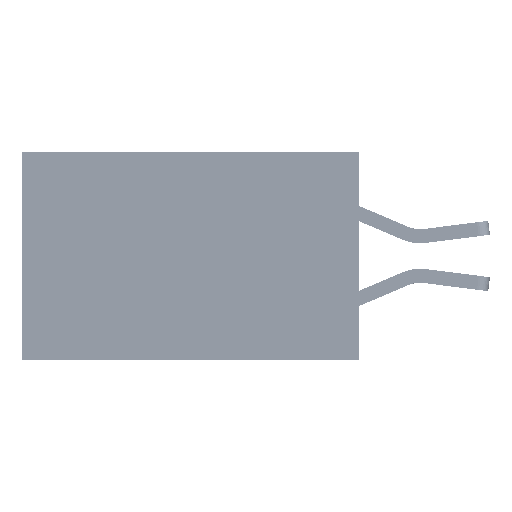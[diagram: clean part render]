
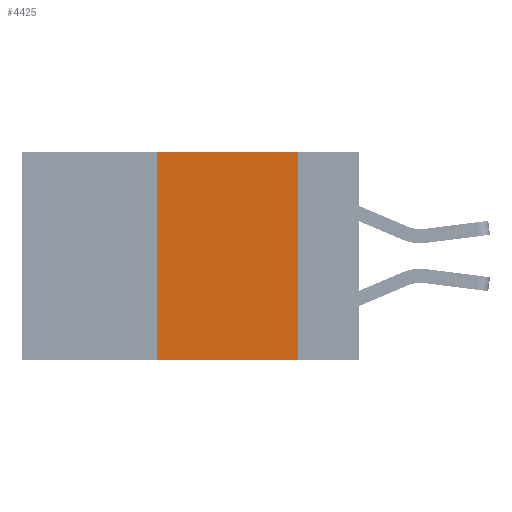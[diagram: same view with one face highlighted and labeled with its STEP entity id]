
A CAD part, left-side view. The second image highlights one B-rep face of the part: STEP entity #4425.
In plain terms, the highlighted planar face has unit normal (-1, 0, 0).
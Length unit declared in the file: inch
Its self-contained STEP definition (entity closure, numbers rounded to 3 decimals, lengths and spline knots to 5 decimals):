
#31 = VERTEX_POINT ( 'NONE', #29388 ) ;
#1272 = CARTESIAN_POINT ( 'NONE',  ( 0., 0.6, -0.37 ) ) ;
#2855 = CARTESIAN_POINT ( 'NONE',  ( 0., 0.6, 0. ) ) ;
#3001 = CARTESIAN_POINT ( 'NONE',  ( 0., 0.11, 0. ) ) ;
#4425 = ADVANCED_FACE ( 'NONE', ( #19435 ), #7295, .F. ) ;
#5041 = VECTOR ( 'NONE', #14315, 39.37008 ) ;
#5146 = VECTOR ( 'NONE', #39077, 39.37008 ) ;
#7295 = PLANE ( 'NONE',  #18443 ) ;
#7898 = EDGE_CURVE ( 'NONE', #31, #11036, #17348, .T. ) ;
#11036 = VERTEX_POINT ( 'NONE', #31494 ) ;
#11077 = ORIENTED_EDGE ( 'NONE', *, *, #44065, .F. ) ;
#12180 = VERTEX_POINT ( 'NONE', #38484 ) ;
#13363 = VERTEX_POINT ( 'NONE', #28481 ) ;
#14315 = DIRECTION ( 'NONE',  ( 0., -1., 0. ) ) ;
#14658 = EDGE_LOOP ( 'NONE', ( #11077, #18350, #37101, #19642 ) ) ;
#14965 = DIRECTION ( 'NONE',  ( 1., 0., 0. ) ) ;
#15253 = LINE ( 'NONE', #2855, #5041 ) ;
#15363 = LINE ( 'NONE', #16987, #5146 ) ;
#16806 = VECTOR ( 'NONE', #18222, 39.37008 ) ;
#16987 = CARTESIAN_POINT ( 'NONE',  ( 0., 0.36, 0. ) ) ;
#17348 = LINE ( 'NONE', #1272, #27207 ) ;
#18222 = DIRECTION ( 'NONE',  ( 0., 0., -1. ) ) ;
#18350 = ORIENTED_EDGE ( 'NONE', *, *, #42104, .F. ) ;
#18443 = AXIS2_PLACEMENT_3D ( 'NONE', #22281, #14965, #40776 ) ;
#19435 = FACE_OUTER_BOUND ( 'NONE', #14658, .T. ) ;
#19642 = ORIENTED_EDGE ( 'NONE', *, *, #7898, .T. ) ;
#21837 = EDGE_CURVE ( 'NONE', #31, #12180, #15363, .T. ) ;
#22281 = CARTESIAN_POINT ( 'NONE',  ( 0., 0.6, 0. ) ) ;
#27207 = VECTOR ( 'NONE', #42366, 39.37008 ) ;
#28481 = CARTESIAN_POINT ( 'NONE',  ( 0., 0.11, 0. ) ) ;
#29388 = CARTESIAN_POINT ( 'NONE',  ( 0., 0.36, -0.37 ) ) ;
#31494 = CARTESIAN_POINT ( 'NONE',  ( 0., 0.11, -0.37 ) ) ;
#35271 = LINE ( 'NONE', #3001, #16806 ) ;
#37101 = ORIENTED_EDGE ( 'NONE', *, *, #21837, .F. ) ;
#38484 = CARTESIAN_POINT ( 'NONE',  ( 0., 0.36, 0. ) ) ;
#39077 = DIRECTION ( 'NONE',  ( 0., 0., 1. ) ) ;
#40776 = DIRECTION ( 'NONE',  ( 0., 0., -1. ) ) ;
#42104 = EDGE_CURVE ( 'NONE', #12180, #13363, #15253, .T. ) ;
#42366 = DIRECTION ( 'NONE',  ( 0., -1., 0. ) ) ;
#44065 = EDGE_CURVE ( 'NONE', #13363, #11036, #35271, .T. ) ;
